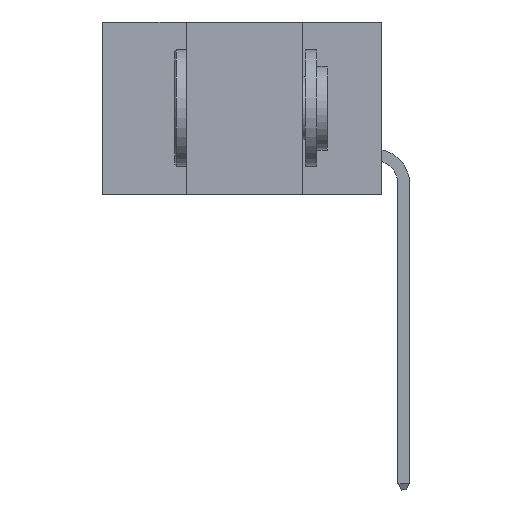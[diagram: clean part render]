
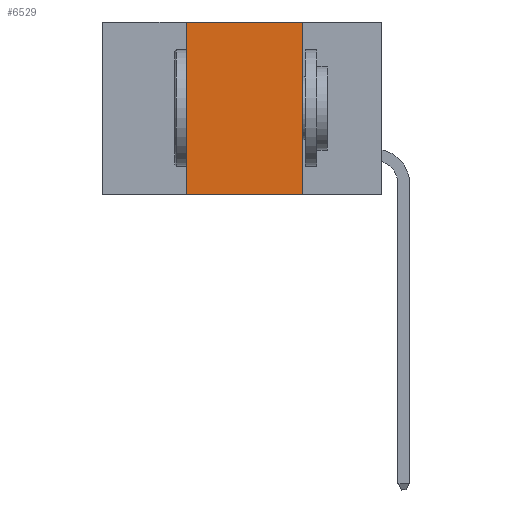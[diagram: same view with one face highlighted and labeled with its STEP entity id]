
A CAD part, left-side view. The second image highlights one B-rep face of the part: STEP entity #6529.
In plain terms, the highlighted planar face has unit normal (-1, 0, 0).
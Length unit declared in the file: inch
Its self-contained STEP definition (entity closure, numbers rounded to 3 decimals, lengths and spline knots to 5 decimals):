
#1086 = EDGE_CURVE ( 'NONE', #22231, #5063, #12427, .T. ) ;
#2128 = CARTESIAN_POINT ( 'NONE',  ( 0., 0.6, 0. ) ) ;
#2228 = PLANE ( 'NONE',  #12455 ) ;
#2248 = ORIENTED_EDGE ( 'NONE', *, *, #1086, .T. ) ;
#5063 = VERTEX_POINT ( 'NONE', #31214 ) ;
#5106 = DIRECTION ( 'NONE',  ( 0., -1., 0. ) ) ;
#6391 = ORIENTED_EDGE ( 'NONE', *, *, #16967, .F. ) ;
#6529 = ADVANCED_FACE ( 'NONE', ( #22724 ), #2228, .F. ) ;
#8913 = DIRECTION ( 'NONE',  ( 0., -1., 0. ) ) ;
#10716 = CARTESIAN_POINT ( 'NONE',  ( 0., 0.17, 0. ) ) ;
#12127 = LINE ( 'NONE', #12778, #14159 ) ;
#12427 = LINE ( 'NONE', #24003, #18780 ) ;
#12455 = AXIS2_PLACEMENT_3D ( 'NONE', #2128, #17181, #32454 ) ;
#12778 = CARTESIAN_POINT ( 'NONE',  ( 0., 0.42, 0. ) ) ;
#13174 = EDGE_LOOP ( 'NONE', ( #16488, #6391, #32821, #2248 ) ) ;
#13268 = DIRECTION ( 'NONE',  ( 0., 0., -1. ) ) ;
#14159 = VECTOR ( 'NONE', #27788, 39.37008 ) ;
#14209 = VERTEX_POINT ( 'NONE', #23462 ) ;
#16488 = ORIENTED_EDGE ( 'NONE', *, *, #21112, .F. ) ;
#16967 = EDGE_CURVE ( 'NONE', #25196, #14209, #29249, .T. ) ;
#17181 = DIRECTION ( 'NONE',  ( 1., 0., 0. ) ) ;
#18780 = VECTOR ( 'NONE', #8913, 39.37008 ) ;
#21112 = EDGE_CURVE ( 'NONE', #14209, #5063, #31359, .T. ) ;
#22055 = EDGE_CURVE ( 'NONE', #22231, #25196, #12127, .T. ) ;
#22149 = CARTESIAN_POINT ( 'NONE',  ( 0., 0.6, 0. ) ) ;
#22231 = VERTEX_POINT ( 'NONE', #23300 ) ;
#22724 = FACE_OUTER_BOUND ( 'NONE', #13174, .T. ) ;
#23300 = CARTESIAN_POINT ( 'NONE',  ( 0., 0.42, -0.37 ) ) ;
#23462 = CARTESIAN_POINT ( 'NONE',  ( 0., 0.17, 0. ) ) ;
#24003 = CARTESIAN_POINT ( 'NONE',  ( 0., 0.6, -0.37 ) ) ;
#24677 = CARTESIAN_POINT ( 'NONE',  ( 0., 0.42, 0. ) ) ;
#25196 = VERTEX_POINT ( 'NONE', #24677 ) ;
#26021 = VECTOR ( 'NONE', #5106, 39.37008 ) ;
#27788 = DIRECTION ( 'NONE',  ( 0., 0., 1. ) ) ;
#29249 = LINE ( 'NONE', #22149, #26021 ) ;
#31214 = CARTESIAN_POINT ( 'NONE',  ( 0., 0.17, -0.37 ) ) ;
#31359 = LINE ( 'NONE', #10716, #32954 ) ;
#32454 = DIRECTION ( 'NONE',  ( 0., 0., -1. ) ) ;
#32821 = ORIENTED_EDGE ( 'NONE', *, *, #22055, .F. ) ;
#32954 = VECTOR ( 'NONE', #13268, 39.37008 ) ;
